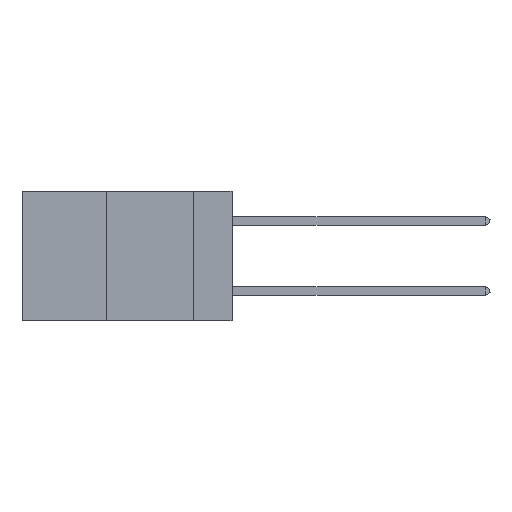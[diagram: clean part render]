
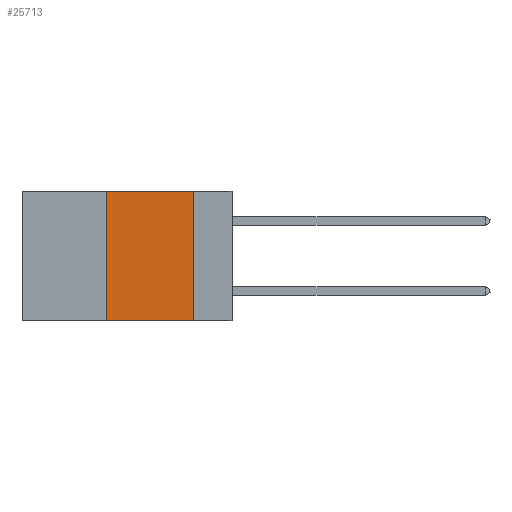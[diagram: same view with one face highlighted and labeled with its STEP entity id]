
A CAD part, left-side view. The second image highlights one B-rep face of the part: STEP entity #25713.
In plain terms, the highlighted planar face has unit normal (-1, 0, 0).
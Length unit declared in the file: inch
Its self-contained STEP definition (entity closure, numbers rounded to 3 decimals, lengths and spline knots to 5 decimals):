
#429 = EDGE_LOOP ( 'NONE', ( #5786, #9308, #8244, #32765 ) ) ;
#1858 = DIRECTION ( 'NONE',  ( 0., 0., 1. ) ) ;
#1910 = CARTESIAN_POINT ( 'NONE',  ( 0., 0.6, -0.37 ) ) ;
#3987 = CARTESIAN_POINT ( 'NONE',  ( 0., 0.11, 0. ) ) ;
#4337 = CARTESIAN_POINT ( 'NONE',  ( 0., 0.36, 0. ) ) ;
#5786 = ORIENTED_EDGE ( 'NONE', *, *, #27009, .F. ) ;
#7537 = LINE ( 'NONE', #3987, #24088 ) ;
#7625 = DIRECTION ( 'NONE',  ( 0., -1., 0. ) ) ;
#7903 = DIRECTION ( 'NONE',  ( 0., -1., 0. ) ) ;
#8244 = ORIENTED_EDGE ( 'NONE', *, *, #16291, .F. ) ;
#8552 = VECTOR ( 'NONE', #7903, 39.37008 ) ;
#9151 = LINE ( 'NONE', #4337, #27484 ) ;
#9308 = ORIENTED_EDGE ( 'NONE', *, *, #25912, .F. ) ;
#10185 = VERTEX_POINT ( 'NONE', #10694 ) ;
#10694 = CARTESIAN_POINT ( 'NONE',  ( 0., 0.36, 0. ) ) ;
#12051 = EDGE_CURVE ( 'NONE', #16666, #25359, #16165, .T. ) ;
#12453 = CARTESIAN_POINT ( 'NONE',  ( 0., 0.11, -0.37 ) ) ;
#13520 = DIRECTION ( 'NONE',  ( 0., 0., -1. ) ) ;
#15100 = VERTEX_POINT ( 'NONE', #27886 ) ;
#16165 = LINE ( 'NONE', #1910, #23289 ) ;
#16291 = EDGE_CURVE ( 'NONE', #16666, #10185, #9151, .T. ) ;
#16666 = VERTEX_POINT ( 'NONE', #36137 ) ;
#22249 = CARTESIAN_POINT ( 'NONE',  ( 0., 0.6, 0. ) ) ;
#23289 = VECTOR ( 'NONE', #7625, 39.37008 ) ;
#24088 = VECTOR ( 'NONE', #26816, 39.37008 ) ;
#25359 = VERTEX_POINT ( 'NONE', #12453 ) ;
#25640 = FACE_OUTER_BOUND ( 'NONE', #429, .T. ) ;
#25713 = ADVANCED_FACE ( 'NONE', ( #25640 ), #30660, .F. ) ;
#25912 = EDGE_CURVE ( 'NONE', #10185, #15100, #35968, .T. ) ;
#26591 = AXIS2_PLACEMENT_3D ( 'NONE', #22249, #33658, #13520 ) ;
#26816 = DIRECTION ( 'NONE',  ( 0., 0., -1. ) ) ;
#27009 = EDGE_CURVE ( 'NONE', #15100, #25359, #7537, .T. ) ;
#27484 = VECTOR ( 'NONE', #1858, 39.37008 ) ;
#27886 = CARTESIAN_POINT ( 'NONE',  ( 0., 0.11, 0. ) ) ;
#30660 = PLANE ( 'NONE',  #26591 ) ;
#32765 = ORIENTED_EDGE ( 'NONE', *, *, #12051, .T. ) ;
#33658 = DIRECTION ( 'NONE',  ( 1., 0., 0. ) ) ;
#35968 = LINE ( 'NONE', #36525, #8552 ) ;
#36137 = CARTESIAN_POINT ( 'NONE',  ( 0., 0.36, -0.37 ) ) ;
#36525 = CARTESIAN_POINT ( 'NONE',  ( 0., 0.6, 0. ) ) ;
